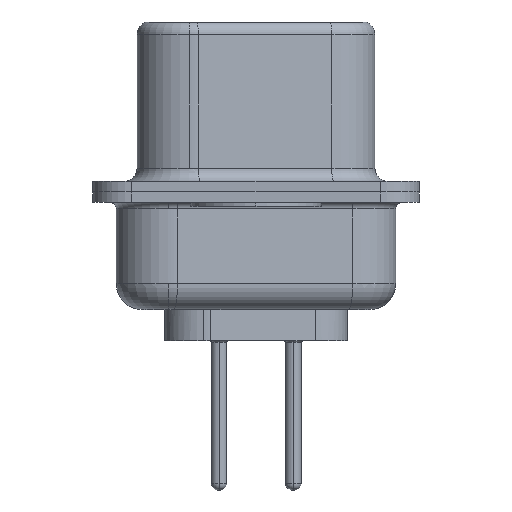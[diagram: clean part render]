
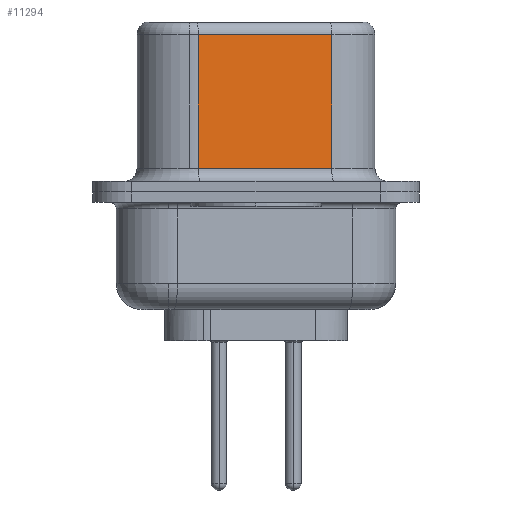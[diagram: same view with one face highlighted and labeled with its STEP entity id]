
A CAD part, left-side view. The second image highlights one B-rep face of the part: STEP entity #11294.
In plain terms, the highlighted planar face has unit normal (-0.985, -0.174, 0).
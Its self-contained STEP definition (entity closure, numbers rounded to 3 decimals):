
#60 = CARTESIAN_POINT ( 'NONE',  ( 4.555, -2.897, 0.9 ) ) ;
#701 = VECTOR ( 'NONE', #5396, 1000. ) ;
#787 = CARTESIAN_POINT ( 'NONE',  ( 3.655, 2.203, 0.9 ) ) ;
#1659 = DIRECTION ( 'NONE',  ( 0.985, 0.174, 0. ) ) ;
#2959 = VECTOR ( 'NONE', #9366, 1000. ) ;
#3364 = DIRECTION ( 'NONE',  ( -0.174, 0.985, 0. ) ) ;
#3663 = ORIENTED_EDGE ( 'NONE', *, *, #9371, .T. ) ;
#3710 = EDGE_CURVE ( 'NONE', #4331, #10446, #5873, .T. ) ;
#4122 = VERTEX_POINT ( 'NONE', #8288 ) ;
#4331 = VERTEX_POINT ( 'NONE', #787 ) ;
#4759 = VERTEX_POINT ( 'NONE', #10076 ) ;
#5276 = EDGE_LOOP ( 'NONE', ( #12831, #3663, #6855, #5732 ) ) ;
#5396 = DIRECTION ( 'NONE',  ( 0., 0., -1. ) ) ;
#5732 = ORIENTED_EDGE ( 'NONE', *, *, #3710, .T. ) ;
#5873 = LINE ( 'NONE', #60, #2959 ) ;
#6855 = ORIENTED_EDGE ( 'NONE', *, *, #13283, .T. ) ;
#7237 = DIRECTION ( 'NONE',  ( 0., 0., -1. ) ) ;
#7828 = LINE ( 'NONE', #9050, #701 ) ;
#8288 = CARTESIAN_POINT ( 'NONE',  ( 3.655, 2.203, 6.02 ) ) ;
#9050 = CARTESIAN_POINT ( 'NONE',  ( 3.655, 2.203, 6.52 ) ) ;
#9201 = CARTESIAN_POINT ( 'NONE',  ( 4.555, -2.897, 0.9 ) ) ;
#9366 = DIRECTION ( 'NONE',  ( 0.174, -0.985, 0. ) ) ;
#9371 = EDGE_CURVE ( 'NONE', #4759, #4122, #10374, .T. ) ;
#9726 = VECTOR ( 'NONE', #7237, 1000. ) ;
#9859 = EDGE_CURVE ( 'NONE', #4759, #10446, #10583, .T. ) ;
#9974 = DIRECTION ( 'NONE',  ( -0.174, 0.985, 0. ) ) ;
#10076 = CARTESIAN_POINT ( 'NONE',  ( 4.555, -2.897, 6.02 ) ) ;
#10251 = VECTOR ( 'NONE', #3364, 1000. ) ;
#10374 = LINE ( 'NONE', #14939, #10251 ) ;
#10446 = VERTEX_POINT ( 'NONE', #9201 ) ;
#10508 = CARTESIAN_POINT ( 'NONE',  ( 4.555, -2.897, 6.52 ) ) ;
#10583 = LINE ( 'NONE', #10508, #9726 ) ;
#11294 = ADVANCED_FACE ( 'NONE', ( #12034 ), #14609, .F. ) ;
#12034 = FACE_OUTER_BOUND ( 'NONE', #5276, .T. ) ;
#12831 = ORIENTED_EDGE ( 'NONE', *, *, #9859, .F. ) ;
#13283 = EDGE_CURVE ( 'NONE', #4122, #4331, #7828, .T. ) ;
#13354 = AXIS2_PLACEMENT_3D ( 'NONE', #14305, #1659, #9974 ) ;
#14305 = CARTESIAN_POINT ( 'NONE',  ( 4.555, -2.897, 6.52 ) ) ;
#14609 = PLANE ( 'NONE',  #13354 ) ;
#14939 = CARTESIAN_POINT ( 'NONE',  ( 4.555, -2.897, 6.02 ) ) ;
